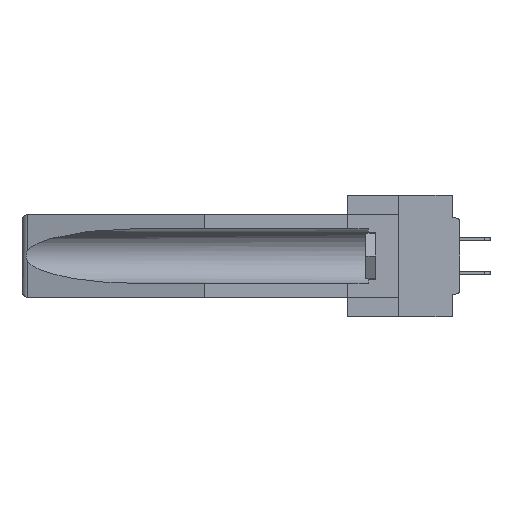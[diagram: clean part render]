
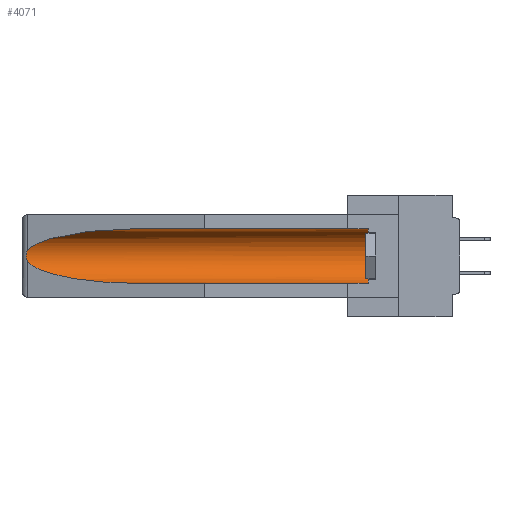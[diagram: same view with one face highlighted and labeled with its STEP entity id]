
A CAD part, left-side view. The second image highlights one B-rep face of the part: STEP entity #4071.
In plain terms, the highlighted cylindrical face has radius 2.857 mm (diameter 5.715 mm), a partial arc.
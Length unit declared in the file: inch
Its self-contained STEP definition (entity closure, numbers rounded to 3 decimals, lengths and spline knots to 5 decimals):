
#240 = CARTESIAN_POINT ( 'NONE',  ( 0.2675, 1.53308, -0.17534 ) ) ;
#359 = EDGE_CURVE ( 'NONE', #7188, #36452, #2551, .T. ) ;
#363 = ORIENTED_EDGE ( 'NONE', *, *, #30329, .T. ) ;
#660 = CARTESIAN_POINT ( 'NONE',  ( 0.26597, 1.52961, -0.15275 ) ) ;
#2469 = EDGE_CURVE ( 'NONE', #15251, #28872, #36121, .T. ) ;
#2551 = LINE ( 'NONE', #42997, #4641 ) ;
#2732 = DIRECTION ( 'NONE',  ( 0., -1., 0. ) ) ;
#2835 = VECTOR ( 'NONE', #25388, 39.37008 ) ;
#3859 = CARTESIAN_POINT ( 'NONE',  ( 0.26537, 1.52718, -0.14972 ) ) ;
#4071 = ADVANCED_FACE ( 'NONE', ( #29750 ), #14158, .F. ) ;
#4641 = VECTOR ( 'NONE', #9934, 39.37008 ) ;
#7188 = VERTEX_POINT ( 'NONE', #24506 ) ;
#8895 = DIRECTION ( 'NONE',  ( 0., 0., 1. ) ) ;
#8973 = ORIENTED_EDGE ( 'NONE', *, *, #2469, .F. ) ;
#9161 = CIRCLE ( 'NONE', #20445, 0.1125 ) ;
#9538 = CARTESIAN_POINT ( 'NONE',  ( 0.26537, 1.52718, -0.14972 ) ) ;
#9765 = DIRECTION ( 'NONE',  ( 0., 1., 0. ) ) ;
#9934 = DIRECTION ( 'NONE',  ( 0., 1., 0. ) ) ;
#9942 = CARTESIAN_POINT ( 'NONE',  ( 0.155, 1.07973, -0.284 ) ) ;
#10811 = VERTEX_POINT ( 'NONE', #42337 ) ;
#10978 = CARTESIAN_POINT ( 'NONE',  ( 0.26537, 1.52718, -0.19328 ) ) ;
#11398 =( BOUNDED_CURVE ( )  B_SPLINE_CURVE ( 3, ( #15424, #19436, #16558, #16852 ),
 .UNSPECIFIED., .F., .F. ) 
 B_SPLINE_CURVE_WITH_KNOTS ( ( 4, 4 ),
 ( 0.1948, 1.5708 ),
 .UNSPECIFIED. ) 
 CURVE ( )  GEOMETRIC_REPRESENTATION_ITEM ( )  RATIONAL_B_SPLINE_CURVE ( ( 1., 0.848, 0.848, 1. ) ) 
 REPRESENTATION_ITEM ( '' )  );
#11604 = EDGE_CURVE ( 'NONE', #10811, #28872, #11398, .T. ) ;
#12314 = EDGE_CURVE ( 'NONE', #36452, #35784, #25801, .T. ) ;
#13488 = CARTESIAN_POINT ( 'NONE',  ( 0.2675, 1.53308, -0.16763 ) ) ;
#14158 = CYLINDRICAL_SURFACE ( 'NONE', #22704, 0.1125 ) ;
#14332 = EDGE_LOOP ( 'NONE', ( #36969, #28012, #16729, #8973, #363, #41457 ) ) ;
#14964 = CARTESIAN_POINT ( 'NONE',  ( 0.155, -0.30754, -0.284 ) ) ;
#15251 = VERTEX_POINT ( 'NONE', #22029 ) ;
#15424 = CARTESIAN_POINT ( 'NONE',  ( 0.26537, 1.52718, -0.19328 ) ) ;
#16558 = CARTESIAN_POINT ( 'NONE',  ( 0.21114, 1.30732, -0.284 ) ) ;
#16729 = ORIENTED_EDGE ( 'NONE', *, *, #11604, .T. ) ;
#16852 = CARTESIAN_POINT ( 'NONE',  ( 0.155, 1.07973, -0.284 ) ) ;
#17373 = CARTESIAN_POINT ( 'NONE',  ( 0.2673, 1.5327, -0.16383 ) ) ;
#19436 = CARTESIAN_POINT ( 'NONE',  ( 0.25451, 1.48313, -0.24835 ) ) ;
#19737 = DIRECTION ( 'NONE',  ( 0., 0., 1. ) ) ;
#20445 = AXIS2_PLACEMENT_3D ( 'NONE', #22697, #2732, #8895 ) ;
#22029 = CARTESIAN_POINT ( 'NONE',  ( 0.155, 0.126, -0.284 ) ) ;
#22697 = CARTESIAN_POINT ( 'NONE',  ( 0.155, 0.126, -0.1715 ) ) ;
#22704 = AXIS2_PLACEMENT_3D ( 'NONE', #29226, #9765, #19737 ) ;
#23935 = CARTESIAN_POINT ( 'NONE',  ( 0.26654, 1.53092, -0.15636 ) ) ;
#24211 = CARTESIAN_POINT ( 'NONE',  ( 0.26655, 1.53094, -0.18657 ) ) ;
#24506 = CARTESIAN_POINT ( 'NONE',  ( 0.155, 0.126, -0.059 ) ) ;
#24618 = CARTESIAN_POINT ( 'NONE',  ( 0.26597, 1.5296, -0.19026 ) ) ;
#25388 = DIRECTION ( 'NONE',  ( 0., 1., 0. ) ) ;
#25786 = CARTESIAN_POINT ( 'NONE',  ( 0.21114, 1.30732, -0.059 ) ) ;
#25801 =( BOUNDED_CURVE ( )  B_SPLINE_CURVE ( 3, ( #32335, #25786, #29008, #9538 ),
 .UNSPECIFIED., .F., .F. ) 
 B_SPLINE_CURVE_WITH_KNOTS ( ( 4, 4 ),
 ( 4.71239, 6.08839 ),
 .UNSPECIFIED. ) 
 CURVE ( )  GEOMETRIC_REPRESENTATION_ITEM ( )  RATIONAL_B_SPLINE_CURVE ( ( 1., 0.848, 0.848, 1. ) ) 
 REPRESENTATION_ITEM ( '' )  );
#27667 = B_SPLINE_CURVE_WITH_KNOTS ( 'NONE', 3,
 ( #3859, #660, #23935, #17373, #13488, #240, #37538, #24211, #24618, #10978 ),
 .UNSPECIFIED., .F., .F.,
 ( 4, 2, 2, 2, 4 ),
 ( 0., 0.00029, 0.00058, 0.00087, 0.00117 ),
 .UNSPECIFIED. ) ;
#27804 = CARTESIAN_POINT ( 'NONE',  ( 0.26537, 1.52718, -0.14972 ) ) ;
#28012 = ORIENTED_EDGE ( 'NONE', *, *, #33205, .T. ) ;
#28342 = CARTESIAN_POINT ( 'NONE',  ( 0.155, 1.07973, -0.059 ) ) ;
#28872 = VERTEX_POINT ( 'NONE', #9942 ) ;
#29008 = CARTESIAN_POINT ( 'NONE',  ( 0.25451, 1.48313, -0.09465 ) ) ;
#29226 = CARTESIAN_POINT ( 'NONE',  ( 0.155, -0.30754, -0.1715 ) ) ;
#29750 = FACE_OUTER_BOUND ( 'NONE', #14332, .T. ) ;
#30329 = EDGE_CURVE ( 'NONE', #15251, #7188, #9161, .T. ) ;
#32335 = CARTESIAN_POINT ( 'NONE',  ( 0.155, 1.07973, -0.059 ) ) ;
#33205 = EDGE_CURVE ( 'NONE', #35784, #10811, #27667, .T. ) ;
#35784 = VERTEX_POINT ( 'NONE', #27804 ) ;
#36121 = LINE ( 'NONE', #14964, #2835 ) ;
#36452 = VERTEX_POINT ( 'NONE', #28342 ) ;
#36969 = ORIENTED_EDGE ( 'NONE', *, *, #12314, .T. ) ;
#37538 = CARTESIAN_POINT ( 'NONE',  ( 0.2673, 1.53269, -0.17917 ) ) ;
#41457 = ORIENTED_EDGE ( 'NONE', *, *, #359, .T. ) ;
#42337 = CARTESIAN_POINT ( 'NONE',  ( 0.26537, 1.52718, -0.19328 ) ) ;
#42997 = CARTESIAN_POINT ( 'NONE',  ( 0.155, -0.30754, -0.059 ) ) ;
